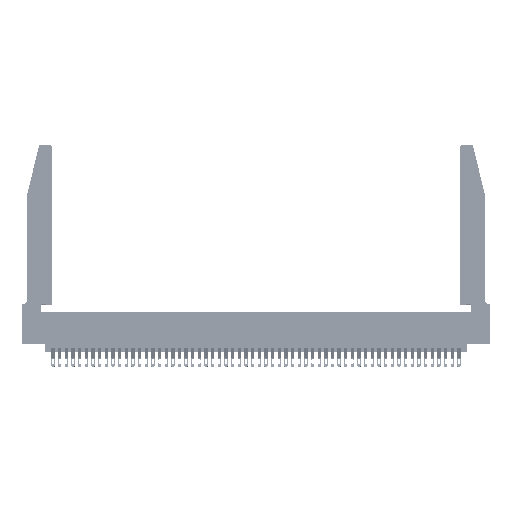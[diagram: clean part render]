
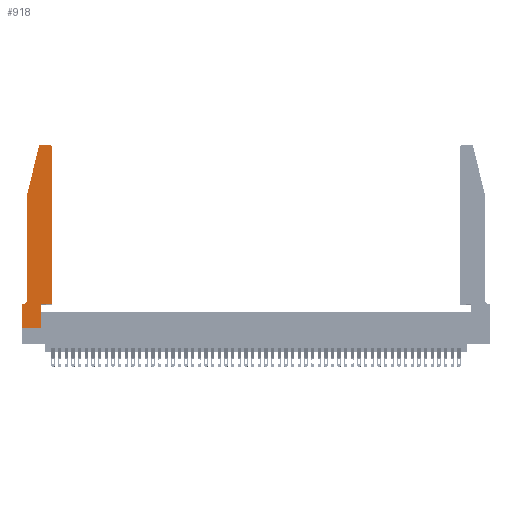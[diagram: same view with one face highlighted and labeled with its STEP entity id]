
A CAD part, top view. The second image highlights one B-rep face of the part: STEP entity #918.
In plain terms, the highlighted planar face has unit normal (0, 0, 1).
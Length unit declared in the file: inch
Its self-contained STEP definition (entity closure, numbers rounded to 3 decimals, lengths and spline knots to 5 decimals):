
#70 = EDGE_CURVE ( 'NONE', #15933, #23846, #16443, .T. ) ;
#173 = FACE_OUTER_BOUND ( 'NONE', #15864, .T. ) ;
#190 = EDGE_CURVE ( 'NONE', #18745, #50549, #10212, .T. ) ;
#330 = DIRECTION ( 'NONE',  ( 1., 0., 0. ) ) ;
#656 = EDGE_CURVE ( 'NONE', #34618, #18745, #20708, .T. ) ;
#719 = DIRECTION ( 'NONE',  ( 0., -1., 0. ) ) ;
#824 = PLANE ( 'NONE',  #37981 ) ;
#895 = EDGE_CURVE ( 'NONE', #36713, #7906, #21287, .T. ) ;
#918 = ADVANCED_FACE ( 'NONE', ( #173 ), #824, .T. ) ;
#1754 = VERTEX_POINT ( 'NONE', #20263 ) ;
#2680 = CARTESIAN_POINT ( 'NONE',  ( 0.0755, 2., 0.37 ) ) ;
#3281 = CARTESIAN_POINT ( 'NONE',  ( 0.0755, 0.35, 0.37 ) ) ;
#3497 = ORIENTED_EDGE ( 'NONE', *, *, #34430, .T. ) ;
#4170 = LINE ( 'NONE', #20727, #24027 ) ;
#4621 = VECTOR ( 'NONE', #19829, 39.37008 ) ;
#4803 = CARTESIAN_POINT ( 'NONE',  ( 0.4205, 2.72, 0.37 ) ) ;
#4820 = CIRCLE ( 'NONE', #45423, 0.03 ) ;
#4966 = CIRCLE ( 'NONE', #39889, 0.07 ) ;
#5191 = CARTESIAN_POINT ( 'NONE',  ( 0., 0., 0.37 ) ) ;
#6641 = LINE ( 'NONE', #2680, #36984 ) ;
#7234 = ORIENTED_EDGE ( 'NONE', *, *, #18600, .T. ) ;
#7906 = VERTEX_POINT ( 'NONE', #38963 ) ;
#7991 = CARTESIAN_POINT ( 'NONE',  ( 0.2605, 2.75, 0.37 ) ) ;
#8488 = ORIENTED_EDGE ( 'NONE', *, *, #895, .T. ) ;
#8503 = ORIENTED_EDGE ( 'NONE', *, *, #70, .T. ) ;
#8763 = DIRECTION ( 'NONE',  ( 0., 1., 0. ) ) ;
#8818 = EDGE_CURVE ( 'NONE', #15786, #30059, #4170, .T. ) ;
#8841 = DIRECTION ( 'NONE',  ( 1., 0., 0. ) ) ;
#9127 = VERTEX_POINT ( 'NONE', #18646 ) ;
#9530 = DIRECTION ( 'NONE',  ( 0., 0., -1. ) ) ;
#9885 = LINE ( 'NONE', #5191, #30935 ) ;
#10212 = LINE ( 'NONE', #20511, #19527 ) ;
#11803 = VECTOR ( 'NONE', #8763, 39.37008 ) ;
#12549 = CARTESIAN_POINT ( 'NONE',  ( 0.284, 2.72, 0.37 ) ) ;
#12804 = DIRECTION ( 'NONE',  ( 1., 0., 0. ) ) ;
#13404 = CARTESIAN_POINT ( 'NONE',  ( 0.25487, 2.72718, 0.37 ) ) ;
#15756 = EDGE_CURVE ( 'NONE', #30059, #9127, #41538, .T. ) ;
#15786 = VERTEX_POINT ( 'NONE', #16335 ) ;
#15864 = EDGE_LOOP ( 'NONE', ( #27639, #3497, #7234, #8503, #42523, #43749, #43168, #33912, #15924, #17133, #48006, #8488 ) ) ;
#15915 = EDGE_CURVE ( 'NONE', #23846, #34618, #4966, .T. ) ;
#15924 = ORIENTED_EDGE ( 'NONE', *, *, #8818, .T. ) ;
#15933 = VERTEX_POINT ( 'NONE', #29227 ) ;
#16168 = CARTESIAN_POINT ( 'NONE',  ( 0.4505, 0.35, 0.37 ) ) ;
#16335 = CARTESIAN_POINT ( 'NONE',  ( 0.2865, 0., 0.37 ) ) ;
#16443 = LINE ( 'NONE', #39528, #4621 ) ;
#16533 = DIRECTION ( 'NONE',  ( 1., 0., 0. ) ) ;
#17133 = ORIENTED_EDGE ( 'NONE', *, *, #15756, .T. ) ;
#18600 = EDGE_CURVE ( 'NONE', #36429, #15933, #6641, .T. ) ;
#18646 = CARTESIAN_POINT ( 'NONE',  ( 0.4505, 0.35, 0.37 ) ) ;
#18745 = VERTEX_POINT ( 'NONE', #31089 ) ;
#19527 = VECTOR ( 'NONE', #719, 39.37008 ) ;
#19829 = DIRECTION ( 'NONE',  ( 0., -1., 0. ) ) ;
#20263 = CARTESIAN_POINT ( 'NONE',  ( 0.284, 2.75, 0.37 ) ) ;
#20511 = CARTESIAN_POINT ( 'NONE',  ( 0., 0., 0.37 ) ) ;
#20708 = LINE ( 'NONE', #3281, #40485 ) ;
#20727 = CARTESIAN_POINT ( 'NONE',  ( 0.2865, 0.35, 0.37 ) ) ;
#21287 = CIRCLE ( 'NONE', #30015, 0.03 ) ;
#22328 = LINE ( 'NONE', #48109, #11803 ) ;
#23064 = DIRECTION ( 'NONE',  ( -1., 0., 0. ) ) ;
#23846 = VERTEX_POINT ( 'NONE', #24775 ) ;
#24027 = VECTOR ( 'NONE', #28468, 39.37008 ) ;
#24566 = CARTESIAN_POINT ( 'NONE',  ( 0., 0.35, 0.37 ) ) ;
#24775 = CARTESIAN_POINT ( 'NONE',  ( 0.0755, 0.42, 0.37 ) ) ;
#26416 = DIRECTION ( 'NONE',  ( -0.239, -0.971, 0. ) ) ;
#27639 = ORIENTED_EDGE ( 'NONE', *, *, #28895, .T. ) ;
#27788 = CARTESIAN_POINT ( 'NONE',  ( 0., 0., 0.37 ) ) ;
#28468 = DIRECTION ( 'NONE',  ( 0., 1., 0. ) ) ;
#28895 = EDGE_CURVE ( 'NONE', #7906, #1754, #30985, .T. ) ;
#29227 = CARTESIAN_POINT ( 'NONE',  ( 0.0755, 2., 0.37 ) ) ;
#30015 = AXIS2_PLACEMENT_3D ( 'NONE', #4803, #32518, #8841 ) ;
#30059 = VERTEX_POINT ( 'NONE', #42985 ) ;
#30935 = VECTOR ( 'NONE', #32760, 39.37008 ) ;
#30985 = LINE ( 'NONE', #7991, #49458 ) ;
#31036 = VECTOR ( 'NONE', #330, 39.37008 ) ;
#31089 = CARTESIAN_POINT ( 'NONE',  ( 0., 0.35, 0.37 ) ) ;
#32518 = DIRECTION ( 'NONE',  ( 0., 0., 1. ) ) ;
#32760 = DIRECTION ( 'NONE',  ( 1., 0., 0. ) ) ;
#33228 = CARTESIAN_POINT ( 'NONE',  ( 0.0055, 0.42, 0.37 ) ) ;
#33912 = ORIENTED_EDGE ( 'NONE', *, *, #44939, .T. ) ;
#34430 = EDGE_CURVE ( 'NONE', #1754, #36429, #4820, .T. ) ;
#34618 = VERTEX_POINT ( 'NONE', #41216 ) ;
#34821 = CARTESIAN_POINT ( 'NONE',  ( 0.4505, 2.72, 0.37 ) ) ;
#36429 = VERTEX_POINT ( 'NONE', #13404 ) ;
#36505 = DIRECTION ( 'NONE',  ( 0., 0., 1. ) ) ;
#36713 = VERTEX_POINT ( 'NONE', #34821 ) ;
#36984 = VECTOR ( 'NONE', #26416, 39.37008 ) ;
#37198 = DIRECTION ( 'NONE',  ( -1., 0., 0. ) ) ;
#37981 = AXIS2_PLACEMENT_3D ( 'NONE', #24566, #36505, #12804 ) ;
#38963 = CARTESIAN_POINT ( 'NONE',  ( 0.4205, 2.75, 0.37 ) ) ;
#39528 = CARTESIAN_POINT ( 'NONE',  ( 0.0755, 2., 0.37 ) ) ;
#39889 = AXIS2_PLACEMENT_3D ( 'NONE', #33228, #9530, #37198 ) ;
#40215 = DIRECTION ( 'NONE',  ( 0., 0., 1. ) ) ;
#40485 = VECTOR ( 'NONE', #23064, 39.37008 ) ;
#41216 = CARTESIAN_POINT ( 'NONE',  ( 0.0055, 0.35, 0.37 ) ) ;
#41538 = LINE ( 'NONE', #16168, #31036 ) ;
#42523 = ORIENTED_EDGE ( 'NONE', *, *, #15915, .T. ) ;
#42985 = CARTESIAN_POINT ( 'NONE',  ( 0.2865, 0.35, 0.37 ) ) ;
#43168 = ORIENTED_EDGE ( 'NONE', *, *, #190, .T. ) ;
#43749 = ORIENTED_EDGE ( 'NONE', *, *, #656, .T. ) ;
#44939 = EDGE_CURVE ( 'NONE', #50549, #15786, #9885, .T. ) ;
#45423 = AXIS2_PLACEMENT_3D ( 'NONE', #12549, #40215, #16533 ) ;
#47348 = DIRECTION ( 'NONE',  ( -1., 0., 0. ) ) ;
#48006 = ORIENTED_EDGE ( 'NONE', *, *, #50679, .T. ) ;
#48109 = CARTESIAN_POINT ( 'NONE',  ( 0.4505, 0.35, 0.37 ) ) ;
#49458 = VECTOR ( 'NONE', #47348, 39.37008 ) ;
#50549 = VERTEX_POINT ( 'NONE', #27788 ) ;
#50679 = EDGE_CURVE ( 'NONE', #9127, #36713, #22328, .T. ) ;
